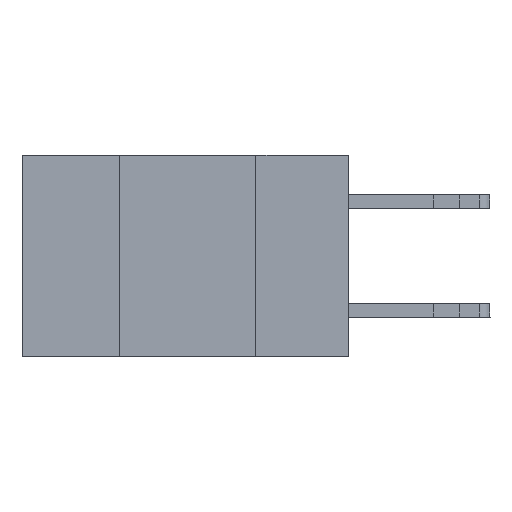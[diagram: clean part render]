
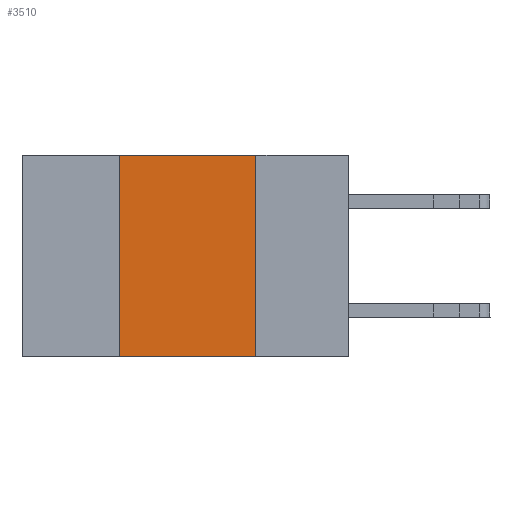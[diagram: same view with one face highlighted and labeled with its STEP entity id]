
A CAD part, left-side view. The second image highlights one B-rep face of the part: STEP entity #3510.
In plain terms, the highlighted planar face has unit normal (-1, 0, 0).
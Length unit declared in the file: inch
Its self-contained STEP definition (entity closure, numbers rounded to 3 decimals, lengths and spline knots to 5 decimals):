
#311 = VERTEX_POINT ( 'NONE', #11376 ) ;
#1169 = DIRECTION ( 'NONE',  ( 0., 0., -1. ) ) ;
#2012 = VECTOR ( 'NONE', #17512, 39.37008 ) ;
#3104 = LINE ( 'NONE', #16226, #16562 ) ;
#3510 = ADVANCED_FACE ( 'NONE', ( #15526 ), #14952, .F. ) ;
#3734 = DIRECTION ( 'NONE',  ( 0., -1., 0. ) ) ;
#3824 = ORIENTED_EDGE ( 'NONE', *, *, #4483, .F. ) ;
#3895 = DIRECTION ( 'NONE',  ( 0., 0., -1. ) ) ;
#3954 = DIRECTION ( 'NONE',  ( 1., 0., 0. ) ) ;
#4238 = EDGE_LOOP ( 'NONE', ( #16538, #15053, #3824, #4563 ) ) ;
#4483 = EDGE_CURVE ( 'NONE', #16222, #9353, #10755, .T. ) ;
#4563 = ORIENTED_EDGE ( 'NONE', *, *, #16097, .T. ) ;
#5501 = LINE ( 'NONE', #14860, #12770 ) ;
#5613 = VECTOR ( 'NONE', #1169, 39.37008 ) ;
#6813 = CARTESIAN_POINT ( 'NONE',  ( 0., 0.6, 0. ) ) ;
#9353 = VERTEX_POINT ( 'NONE', #10023 ) ;
#10008 = CARTESIAN_POINT ( 'NONE',  ( 0., 0.42, -0.37 ) ) ;
#10023 = CARTESIAN_POINT ( 'NONE',  ( 0., 0.42, 0. ) ) ;
#10492 = LINE ( 'NONE', #17527, #5613 ) ;
#10530 = EDGE_CURVE ( 'NONE', #9353, #16289, #3104, .T. ) ;
#10755 = LINE ( 'NONE', #17360, #2012 ) ;
#11119 = CARTESIAN_POINT ( 'NONE',  ( 0., 0.17, 0. ) ) ;
#11376 = CARTESIAN_POINT ( 'NONE',  ( 0., 0.17, -0.37 ) ) ;
#12770 = VECTOR ( 'NONE', #3734, 39.37008 ) ;
#13273 = EDGE_CURVE ( 'NONE', #16289, #311, #10492, .T. ) ;
#14860 = CARTESIAN_POINT ( 'NONE',  ( 0., 0.6, -0.37 ) ) ;
#14952 = PLANE ( 'NONE',  #16879 ) ;
#15053 = ORIENTED_EDGE ( 'NONE', *, *, #10530, .F. ) ;
#15526 = FACE_OUTER_BOUND ( 'NONE', #4238, .T. ) ;
#16097 = EDGE_CURVE ( 'NONE', #16222, #311, #5501, .T. ) ;
#16222 = VERTEX_POINT ( 'NONE', #10008 ) ;
#16226 = CARTESIAN_POINT ( 'NONE',  ( 0., 0.6, 0. ) ) ;
#16289 = VERTEX_POINT ( 'NONE', #11119 ) ;
#16538 = ORIENTED_EDGE ( 'NONE', *, *, #13273, .F. ) ;
#16562 = VECTOR ( 'NONE', #16571, 39.37008 ) ;
#16571 = DIRECTION ( 'NONE',  ( 0., -1., 0. ) ) ;
#16879 = AXIS2_PLACEMENT_3D ( 'NONE', #6813, #3954, #3895 ) ;
#17360 = CARTESIAN_POINT ( 'NONE',  ( 0., 0.42, 0. ) ) ;
#17512 = DIRECTION ( 'NONE',  ( 0., 0., 1. ) ) ;
#17527 = CARTESIAN_POINT ( 'NONE',  ( 0., 0.17, 0. ) ) ;
